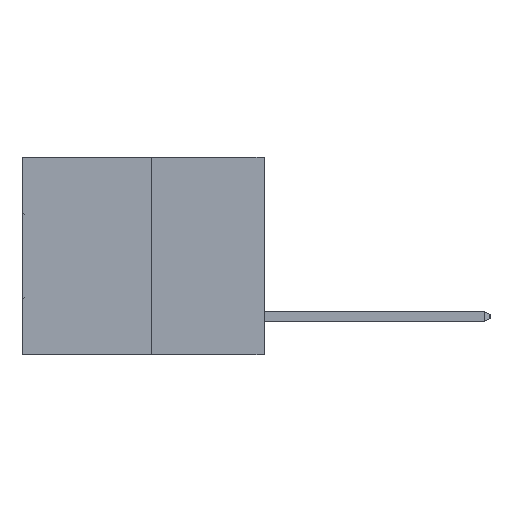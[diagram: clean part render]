
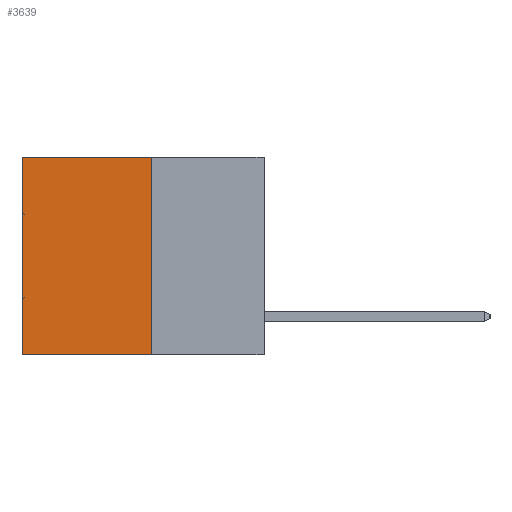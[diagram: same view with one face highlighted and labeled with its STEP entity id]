
A CAD part, left-side view. The second image highlights one B-rep face of the part: STEP entity #3639.
In plain terms, the highlighted planar face has unit normal (-1, 0, 0).
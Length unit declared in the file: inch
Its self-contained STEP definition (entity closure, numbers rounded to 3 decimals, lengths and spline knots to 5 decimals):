
#1305 = VERTEX_POINT ( 'NONE', #26926 ) ;
#1400 = LINE ( 'NONE', #6037, #19509 ) ;
#2143 = DIRECTION ( 'NONE',  ( 1., 0., 0. ) ) ;
#3124 = FACE_OUTER_BOUND ( 'NONE', #8515, .T. ) ;
#3639 = ADVANCED_FACE ( 'NONE', ( #3124 ), #30573, .F. ) ;
#4405 = VERTEX_POINT ( 'NONE', #32883 ) ;
#4448 = VERTEX_POINT ( 'NONE', #15468 ) ;
#6037 = CARTESIAN_POINT ( 'NONE',  ( 0.3165, 0.28, 0. ) ) ;
#7504 = EDGE_CURVE ( 'NONE', #28474, #1305, #22702, .T. ) ;
#8291 = ORIENTED_EDGE ( 'NONE', *, *, #28222, .F. ) ;
#8515 = EDGE_LOOP ( 'NONE', ( #12735, #8291, #19685, #26121 ) ) ;
#11124 = CARTESIAN_POINT ( 'NONE',  ( 0.3165, 0.28, -0.49 ) ) ;
#12735 = ORIENTED_EDGE ( 'NONE', *, *, #16964, .T. ) ;
#13081 = LINE ( 'NONE', #31168, #33248 ) ;
#13397 = DIRECTION ( 'NONE',  ( 0., 1., 0. ) ) ;
#13798 = AXIS2_PLACEMENT_3D ( 'NONE', #27878, #2143, #20145 ) ;
#15468 = CARTESIAN_POINT ( 'NONE',  ( 0.3165, 0.6, -0.49 ) ) ;
#16302 = CARTESIAN_POINT ( 'NONE',  ( 0.3165, 0.28, -0.49 ) ) ;
#16964 = EDGE_CURVE ( 'NONE', #4405, #4448, #13081, .T. ) ;
#19509 = VECTOR ( 'NONE', #24065, 39.37008 ) ;
#19685 = ORIENTED_EDGE ( 'NONE', *, *, #7504, .F. ) ;
#20145 = DIRECTION ( 'NONE',  ( 0., 0., -1. ) ) ;
#20524 = LINE ( 'NONE', #16302, #27508 ) ;
#21335 = DIRECTION ( 'NONE',  ( 0., 0., -1. ) ) ;
#21501 = CARTESIAN_POINT ( 'NONE',  ( 0.3165, 0.28, 0. ) ) ;
#22702 = LINE ( 'NONE', #11124, #28029 ) ;
#22708 = EDGE_CURVE ( 'NONE', #28474, #4405, #1400, .T. ) ;
#24065 = DIRECTION ( 'NONE',  ( 0., 1., 0. ) ) ;
#26121 = ORIENTED_EDGE ( 'NONE', *, *, #22708, .T. ) ;
#26926 = CARTESIAN_POINT ( 'NONE',  ( 0.3165, 0.28, -0.49 ) ) ;
#27226 = DIRECTION ( 'NONE',  ( 0., 0., -1. ) ) ;
#27508 = VECTOR ( 'NONE', #13397, 39.37008 ) ;
#27878 = CARTESIAN_POINT ( 'NONE',  ( 0.3165, 0.28, -0.49 ) ) ;
#28029 = VECTOR ( 'NONE', #21335, 39.37008 ) ;
#28222 = EDGE_CURVE ( 'NONE', #1305, #4448, #20524, .T. ) ;
#28474 = VERTEX_POINT ( 'NONE', #21501 ) ;
#30573 = PLANE ( 'NONE',  #13798 ) ;
#31168 = CARTESIAN_POINT ( 'NONE',  ( 0.3165, 0.6, -0.49 ) ) ;
#32883 = CARTESIAN_POINT ( 'NONE',  ( 0.3165, 0.6, 0. ) ) ;
#33248 = VECTOR ( 'NONE', #27226, 39.37008 ) ;
